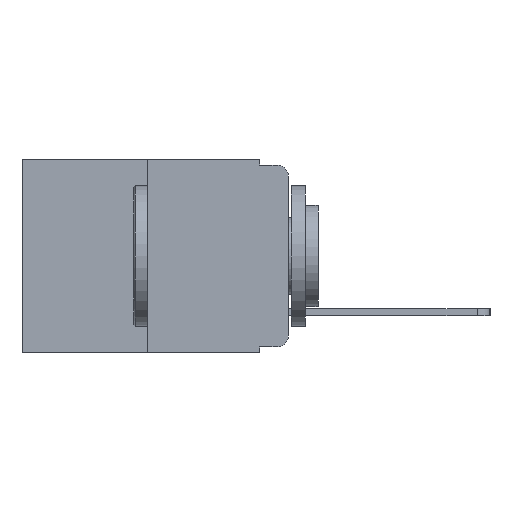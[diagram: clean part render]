
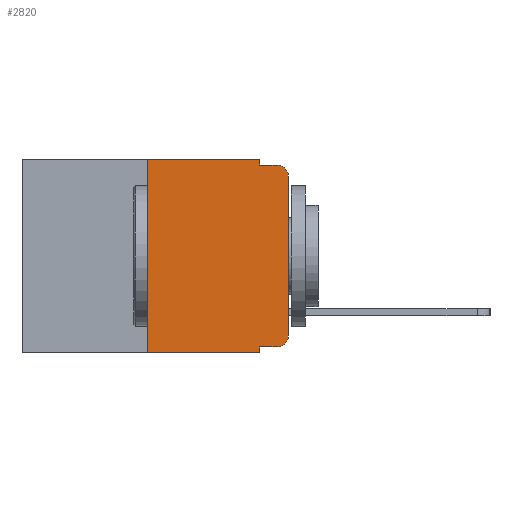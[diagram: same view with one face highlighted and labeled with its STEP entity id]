
A CAD part, left-side view. The second image highlights one B-rep face of the part: STEP entity #2820.
In plain terms, the highlighted planar face has unit normal (-1, 0, 0).
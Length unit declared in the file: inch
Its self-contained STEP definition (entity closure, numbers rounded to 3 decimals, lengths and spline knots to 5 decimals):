
#352 = DIRECTION ( 'NONE',  ( 1., 0., 0. ) ) ;
#452 = DIRECTION ( 'NONE',  ( 0., 0., 1. ) ) ;
#462 = DIRECTION ( 'NONE',  ( 0., -1., 0. ) ) ;
#533 = VERTEX_POINT ( 'NONE', #5140 ) ;
#738 = CARTESIAN_POINT ( 'NONE',  ( 0., 0.02, -0.03 ) ) ;
#793 = ORIENTED_EDGE ( 'NONE', *, *, #2938, .F. ) ;
#843 = CARTESIAN_POINT ( 'NONE',  ( 0., 0.02, -0.313 ) ) ;
#1018 = ORIENTED_EDGE ( 'NONE', *, *, #8048, .T. ) ;
#1099 = ORIENTED_EDGE ( 'NONE', *, *, #7573, .T. ) ;
#1161 = DIRECTION ( 'NONE',  ( 0., 0., -1. ) ) ;
#1323 = DIRECTION ( 'NONE',  ( 0., 0., -1. ) ) ;
#1450 = ORIENTED_EDGE ( 'NONE', *, *, #2049, .F. ) ;
#1577 = EDGE_CURVE ( 'NONE', #3574, #11184, #8324, .T. ) ;
#1725 = DIRECTION ( 'NONE',  ( 0., 0., -1. ) ) ;
#1742 = VERTEX_POINT ( 'NONE', #11729 ) ;
#1874 = CARTESIAN_POINT ( 'NONE',  ( 0., 0.051, -0.333 ) ) ;
#1898 = EDGE_CURVE ( 'NONE', #533, #3574, #9193, .T. ) ;
#2049 = EDGE_CURVE ( 'NONE', #7149, #533, #11254, .T. ) ;
#2304 = LINE ( 'NONE', #5500, #7144 ) ;
#2369 = CARTESIAN_POINT ( 'NONE',  ( 0., 0.051, -0.01 ) ) ;
#2398 = EDGE_CURVE ( 'NONE', #6457, #4758, #12087, .T. ) ;
#2554 = FACE_OUTER_BOUND ( 'NONE', #11752, .T. ) ;
#2600 = LINE ( 'NONE', #4347, #9667 ) ;
#2606 = ORIENTED_EDGE ( 'NONE', *, *, #12019, .T. ) ;
#2820 = ADVANCED_FACE ( 'NONE', ( #2554 ), #11868, .F. ) ;
#2853 = CARTESIAN_POINT ( 'NONE',  ( 0., 0.051, 0. ) ) ;
#2938 = EDGE_CURVE ( 'NONE', #7696, #1742, #7406, .T. ) ;
#3240 = CARTESIAN_POINT ( 'NONE',  ( 0., 0., -0.03 ) ) ;
#3376 = CIRCLE ( 'NONE', #4974, 0.02 ) ;
#3523 = ORIENTED_EDGE ( 'NONE', *, *, #5863, .F. ) ;
#3574 = VERTEX_POINT ( 'NONE', #9735 ) ;
#3585 = CARTESIAN_POINT ( 'NONE',  ( 0., 0.25, -0.343 ) ) ;
#3791 = VECTOR ( 'NONE', #1161, 39.37008 ) ;
#4052 = AXIS2_PLACEMENT_3D ( 'NONE', #843, #8531, #8463 ) ;
#4329 = CARTESIAN_POINT ( 'NONE',  ( 0., 0.473, 0. ) ) ;
#4347 = CARTESIAN_POINT ( 'NONE',  ( 0., 0.473, -0.343 ) ) ;
#4423 = DIRECTION ( 'NONE',  ( 0., -1., 0. ) ) ;
#4534 = DIRECTION ( 'NONE',  ( 0., -1., 0. ) ) ;
#4558 = CARTESIAN_POINT ( 'NONE',  ( 0., 0.051, 0. ) ) ;
#4586 = ORIENTED_EDGE ( 'NONE', *, *, #1577, .F. ) ;
#4618 = DIRECTION ( 'NONE',  ( 0., 0., -1. ) ) ;
#4758 = VERTEX_POINT ( 'NONE', #8304 ) ;
#4974 = AXIS2_PLACEMENT_3D ( 'NONE', #738, #7506, #1725 ) ;
#5110 = VERTEX_POINT ( 'NONE', #9733 ) ;
#5140 = CARTESIAN_POINT ( 'NONE',  ( 0., 0.25, 0. ) ) ;
#5312 = CARTESIAN_POINT ( 'NONE',  ( 0., 0.25, 0. ) ) ;
#5500 = CARTESIAN_POINT ( 'NONE',  ( 0., 0.051, -0.333 ) ) ;
#5689 = ORIENTED_EDGE ( 'NONE', *, *, #11247, .T. ) ;
#5863 = EDGE_CURVE ( 'NONE', #11184, #5110, #9144, .T. ) ;
#5919 = VECTOR ( 'NONE', #7328, 39.37008 ) ;
#6457 = VERTEX_POINT ( 'NONE', #9057 ) ;
#6587 = VECTOR ( 'NONE', #462, 39.37008 ) ;
#6642 = VECTOR ( 'NONE', #4423, 39.37008 ) ;
#6831 = LINE ( 'NONE', #7212, #11543 ) ;
#6976 = ORIENTED_EDGE ( 'NONE', *, *, #2398, .T. ) ;
#7144 = VECTOR ( 'NONE', #4534, 39.37008 ) ;
#7149 = VERTEX_POINT ( 'NONE', #3585 ) ;
#7212 = CARTESIAN_POINT ( 'NONE',  ( 0., 0., 0. ) ) ;
#7328 = DIRECTION ( 'NONE',  ( 0., 0., 1. ) ) ;
#7406 = LINE ( 'NONE', #2853, #3791 ) ;
#7506 = DIRECTION ( 'NONE',  ( -1., 0., 0. ) ) ;
#7573 = EDGE_CURVE ( 'NONE', #7696, #6457, #2304, .T. ) ;
#7696 = VERTEX_POINT ( 'NONE', #1874 ) ;
#8048 = EDGE_CURVE ( 'NONE', #4758, #8534, #6831, .T. ) ;
#8304 = CARTESIAN_POINT ( 'NONE',  ( 0., 0., -0.313 ) ) ;
#8324 = LINE ( 'NONE', #4558, #9926 ) ;
#8463 = DIRECTION ( 'NONE',  ( 0., 0., -1. ) ) ;
#8531 = DIRECTION ( 'NONE',  ( -1., 0., 0. ) ) ;
#8534 = VERTEX_POINT ( 'NONE', #3240 ) ;
#9052 = CARTESIAN_POINT ( 'NONE',  ( 0., 0.051, -0.01 ) ) ;
#9057 = CARTESIAN_POINT ( 'NONE',  ( 0., 0.02, -0.333 ) ) ;
#9091 = CARTESIAN_POINT ( 'NONE',  ( 0., 0.473, 0. ) ) ;
#9144 = LINE ( 'NONE', #2369, #6587 ) ;
#9193 = LINE ( 'NONE', #9091, #6642 ) ;
#9223 = ORIENTED_EDGE ( 'NONE', *, *, #1898, .F. ) ;
#9667 = VECTOR ( 'NONE', #10964, 39.37008 ) ;
#9733 = CARTESIAN_POINT ( 'NONE',  ( 0., 0.02, -0.01 ) ) ;
#9735 = CARTESIAN_POINT ( 'NONE',  ( 0., 0.051, 0. ) ) ;
#9926 = VECTOR ( 'NONE', #4618, 39.37008 ) ;
#10853 = AXIS2_PLACEMENT_3D ( 'NONE', #4329, #352, #1323 ) ;
#10964 = DIRECTION ( 'NONE',  ( 0., -1., 0. ) ) ;
#11184 = VERTEX_POINT ( 'NONE', #9052 ) ;
#11247 = EDGE_CURVE ( 'NONE', #7149, #1742, #2600, .T. ) ;
#11254 = LINE ( 'NONE', #5312, #5919 ) ;
#11543 = VECTOR ( 'NONE', #452, 39.37008 ) ;
#11729 = CARTESIAN_POINT ( 'NONE',  ( 0., 0.051, -0.343 ) ) ;
#11752 = EDGE_LOOP ( 'NONE', ( #1018, #2606, #3523, #4586, #9223, #1450, #5689, #793, #1099, #6976 ) ) ;
#11868 = PLANE ( 'NONE',  #10853 ) ;
#12019 = EDGE_CURVE ( 'NONE', #8534, #5110, #3376, .T. ) ;
#12087 = CIRCLE ( 'NONE', #4052, 0.02 ) ;
